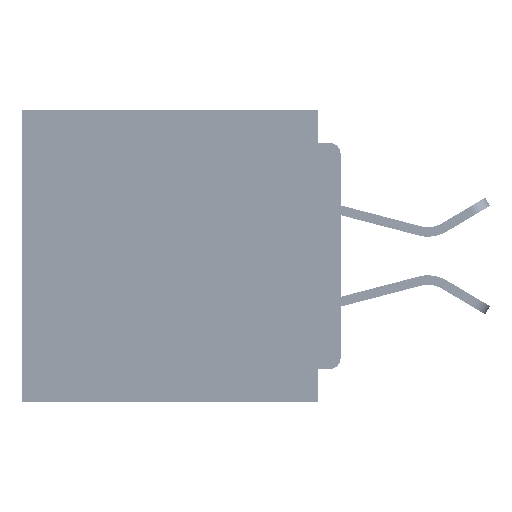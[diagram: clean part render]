
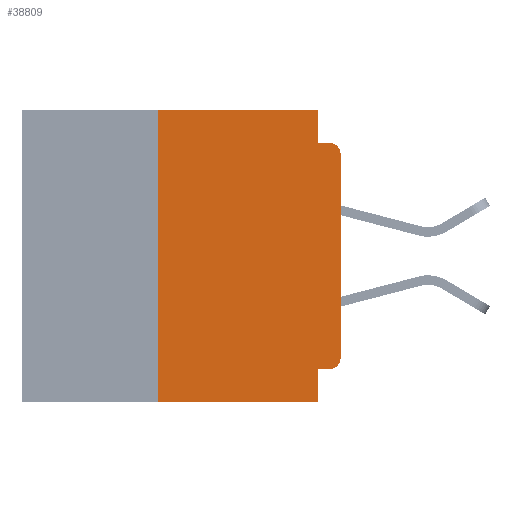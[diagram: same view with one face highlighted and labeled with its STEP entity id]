
A CAD part, left-side view. The second image highlights one B-rep face of the part: STEP entity #38809.
In plain terms, the highlighted planar face has unit normal (-1, 0, 0).
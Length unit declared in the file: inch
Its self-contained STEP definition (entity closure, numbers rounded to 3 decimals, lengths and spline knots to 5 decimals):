
#8 = DIRECTION ( 'NONE',  ( 0., -1., 0. ) ) ;
#331 = EDGE_CURVE ( 'NONE', #55111, #49715, #66854, .T. ) ;
#508 = CARTESIAN_POINT ( 'NONE',  ( 0., 0.015, -0.045 ) ) ;
#979 = CARTESIAN_POINT ( 'NONE',  ( 0., 0.031, -0.355 ) ) ;
#1227 = LINE ( 'NONE', #49852, #27612 ) ;
#2107 = VERTEX_POINT ( 'NONE', #979 ) ;
#2333 = CARTESIAN_POINT ( 'NONE',  ( 0., 0.437, 0. ) ) ;
#3485 = CARTESIAN_POINT ( 'NONE',  ( 0., 0.031, -0.4 ) ) ;
#4943 = DIRECTION ( 'NONE',  ( 0., -1., 0. ) ) ;
#5322 = CARTESIAN_POINT ( 'NONE',  ( 0., 0., -0.045 ) ) ;
#6221 = CARTESIAN_POINT ( 'NONE',  ( 0., 0., -0.355 ) ) ;
#6366 = EDGE_CURVE ( 'NONE', #55111, #2107, #28825, .T. ) ;
#7439 = ORIENTED_EDGE ( 'NONE', *, *, #54021, .T. ) ;
#7884 = EDGE_CURVE ( 'NONE', #30985, #64178, #53073, .T. ) ;
#8003 = VERTEX_POINT ( 'NONE', #3485 ) ;
#8836 = VECTOR ( 'NONE', #4943, 39.37008 ) ;
#11773 = CARTESIAN_POINT ( 'NONE',  ( 0., 0., -0.06 ) ) ;
#13755 = CARTESIAN_POINT ( 'NONE',  ( 0., 0.25, -0.4 ) ) ;
#15303 = VERTEX_POINT ( 'NONE', #11773 ) ;
#15718 = EDGE_CURVE ( 'NONE', #2107, #8003, #38071, .T. ) ;
#16279 = CIRCLE ( 'NONE', #50012, 0.015 ) ;
#16507 = CARTESIAN_POINT ( 'NONE',  ( 0., 0.015, -0.06 ) ) ;
#16914 = CARTESIAN_POINT ( 'NONE',  ( 0., 0.437, 0. ) ) ;
#19926 = AXIS2_PLACEMENT_3D ( 'NONE', #16914, #53473, #22189 ) ;
#20198 = CARTESIAN_POINT ( 'NONE',  ( 0., 0.25, 0. ) ) ;
#20297 = VECTOR ( 'NONE', #27443, 39.37008 ) ;
#21349 = VERTEX_POINT ( 'NONE', #13755 ) ;
#21768 = DIRECTION ( 'NONE',  ( 0., 0., -1. ) ) ;
#21829 = VECTOR ( 'NONE', #8, 39.37008 ) ;
#22189 = DIRECTION ( 'NONE',  ( 0., 0., -1. ) ) ;
#23766 = EDGE_CURVE ( 'NONE', #64178, #55231, #1227, .T. ) ;
#25984 = DIRECTION ( 'NONE',  ( 0., 0., -1. ) ) ;
#26020 = CARTESIAN_POINT ( 'NONE',  ( 0., 0.031, -0.045 ) ) ;
#27174 = VECTOR ( 'NONE', #53417, 39.37008 ) ;
#27199 = ORIENTED_EDGE ( 'NONE', *, *, #23766, .F. ) ;
#27443 = DIRECTION ( 'NONE',  ( 0., 0., 1. ) ) ;
#27558 = LINE ( 'NONE', #32870, #38158 ) ;
#27612 = VECTOR ( 'NONE', #55079, 39.37008 ) ;
#28020 = EDGE_CURVE ( 'NONE', #55231, #34790, #49645, .T. ) ;
#28196 = EDGE_CURVE ( 'NONE', #21349, #30985, #27558, .T. ) ;
#28825 = LINE ( 'NONE', #6221, #27174 ) ;
#30985 = VERTEX_POINT ( 'NONE', #20198 ) ;
#31160 = CARTESIAN_POINT ( 'NONE',  ( 0., 0.437, -0.4 ) ) ;
#32870 = CARTESIAN_POINT ( 'NONE',  ( 0., 0.25, -0.4 ) ) ;
#32873 = ORIENTED_EDGE ( 'NONE', *, *, #54719, .T. ) ;
#34524 = ORIENTED_EDGE ( 'NONE', *, *, #54143, .T. ) ;
#34790 = VERTEX_POINT ( 'NONE', #508 ) ;
#35626 = CARTESIAN_POINT ( 'NONE',  ( 0., 0.015, -0.355 ) ) ;
#36193 = ORIENTED_EDGE ( 'NONE', *, *, #28020, .F. ) ;
#37725 = PLANE ( 'NONE',  #19926 ) ;
#38071 = LINE ( 'NONE', #41477, #65801 ) ;
#38158 = VECTOR ( 'NONE', #48669, 39.37008 ) ;
#38387 = CARTESIAN_POINT ( 'NONE',  ( 0., 0.015, -0.34 ) ) ;
#38809 = ADVANCED_FACE ( 'NONE', ( #39807 ), #37725, .F. ) ;
#39076 = DIRECTION ( 'NONE',  ( 0., -1., 0. ) ) ;
#39807 = FACE_OUTER_BOUND ( 'NONE', #53121, .T. ) ;
#41066 = ORIENTED_EDGE ( 'NONE', *, *, #7884, .F. ) ;
#41477 = CARTESIAN_POINT ( 'NONE',  ( 0., 0.031, -0.4 ) ) ;
#42233 = AXIS2_PLACEMENT_3D ( 'NONE', #38387, #45194, #44957 ) ;
#44957 = DIRECTION ( 'NONE',  ( 0., 0., -1. ) ) ;
#45194 = DIRECTION ( 'NONE',  ( -1., 0., 0. ) ) ;
#47620 = CARTESIAN_POINT ( 'NONE',  ( 0., 0., -0.34 ) ) ;
#47625 = ORIENTED_EDGE ( 'NONE', *, *, #28196, .F. ) ;
#48669 = DIRECTION ( 'NONE',  ( 0., 0., 1. ) ) ;
#49645 = LINE ( 'NONE', #5322, #21829 ) ;
#49715 = VERTEX_POINT ( 'NONE', #47620 ) ;
#49852 = CARTESIAN_POINT ( 'NONE',  ( 0., 0.031, 0. ) ) ;
#50012 = AXIS2_PLACEMENT_3D ( 'NONE', #16507, #53058, #21768 ) ;
#51457 = VECTOR ( 'NONE', #39076, 39.37008 ) ;
#53058 = DIRECTION ( 'NONE',  ( -1., 0., 0. ) ) ;
#53073 = LINE ( 'NONE', #2333, #51457 ) ;
#53121 = EDGE_LOOP ( 'NONE', ( #32873, #34524, #36193, #27199, #41066, #47625, #7439, #63132, #55810, #57439 ) ) ;
#53417 = DIRECTION ( 'NONE',  ( 0., 1., 0. ) ) ;
#53473 = DIRECTION ( 'NONE',  ( 1., 0., 0. ) ) ;
#53769 = CARTESIAN_POINT ( 'NONE',  ( 0., 0.031, 0. ) ) ;
#54021 = EDGE_CURVE ( 'NONE', #21349, #8003, #64485, .T. ) ;
#54143 = EDGE_CURVE ( 'NONE', #15303, #34790, #16279, .T. ) ;
#54719 = EDGE_CURVE ( 'NONE', #49715, #15303, #60297, .T. ) ;
#55079 = DIRECTION ( 'NONE',  ( 0., 0., -1. ) ) ;
#55111 = VERTEX_POINT ( 'NONE', #35626 ) ;
#55231 = VERTEX_POINT ( 'NONE', #26020 ) ;
#55810 = ORIENTED_EDGE ( 'NONE', *, *, #6366, .F. ) ;
#57439 = ORIENTED_EDGE ( 'NONE', *, *, #331, .T. ) ;
#58689 = CARTESIAN_POINT ( 'NONE',  ( 0., 0., 0. ) ) ;
#60297 = LINE ( 'NONE', #58689, #20297 ) ;
#63132 = ORIENTED_EDGE ( 'NONE', *, *, #15718, .F. ) ;
#64178 = VERTEX_POINT ( 'NONE', #53769 ) ;
#64485 = LINE ( 'NONE', #31160, #8836 ) ;
#65801 = VECTOR ( 'NONE', #25984, 39.37008 ) ;
#66854 = CIRCLE ( 'NONE', #42233, 0.015 ) ;
